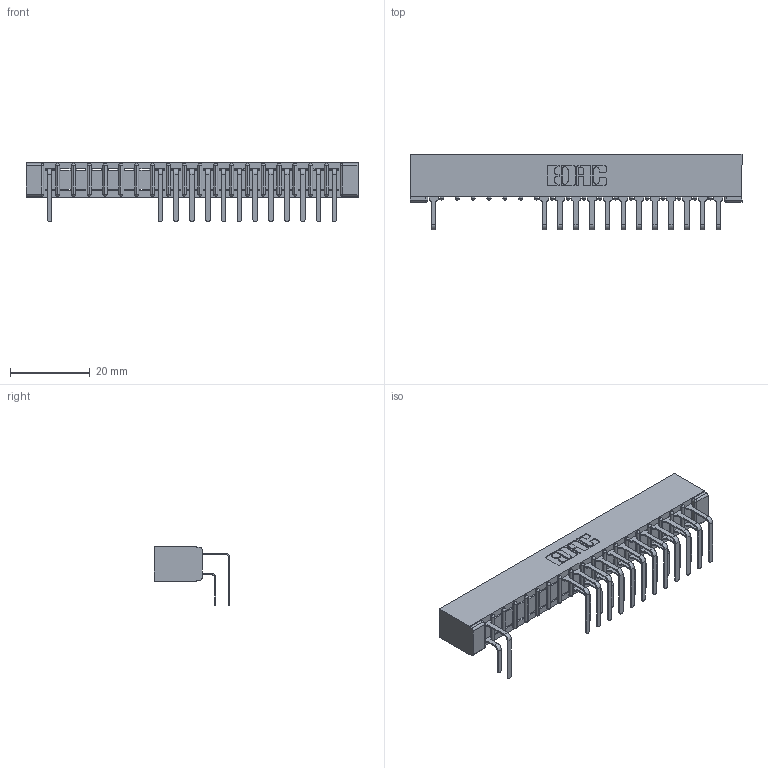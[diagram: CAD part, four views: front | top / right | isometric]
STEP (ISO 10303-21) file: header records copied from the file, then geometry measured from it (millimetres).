
FILE_DESCRIPTION (( 'STEP AP203' ), '1' );
FILE_NAME ('307-019-558-101.STEP', '2018-08-04T00:05:55', ( '' ), ( '' ), 'SwSTEP 2.0', 'SolidWorks 2016', '' );
FILE_SCHEMA (( 'CONFIG_CONTROL_DESIGN' ));
Length unit declared in the file: inch
Products named in the file (4): 307-290-001_558 559 - 1 (Single); 307-290-001_558 - 2 (Single); 307-019-558-101; 307 Part_No Mounting Lugs
Assembly tree (26 placements, depth 2):
  307-019-558-101
    307 Part_No Mounting Lugs
    307-290-001_558 559 - 1 (Single)  x12
    307-290-001_558 - 2 (Single)  x13
Bounding box: 83.16 x 18.96 x 14.81 mm (x, y, z)
Volume: 5617.1 mm3; surface area: 9875.4 mm2
Topology: 26 solids, 26 shells, 1510 faces, 4265 edges, 2754 vertices
Faces by surface type: plane 969, cylinder 501, sphere 40
Entity records: 20485 total; most frequent: CARTESIAN_POINT 3412, ORIENTED_EDGE 3390, DIRECTION 3337, EDGE_CURVE 1695, LINE 1291, VECTOR 1291, VERTEX_POINT 1098, AXIS2_PLACEMENT_3D 1023
